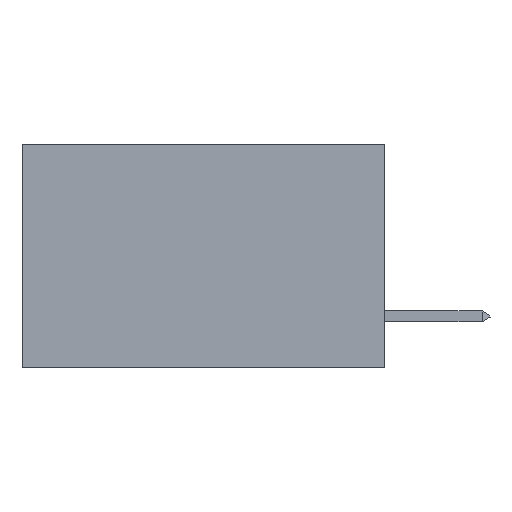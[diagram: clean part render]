
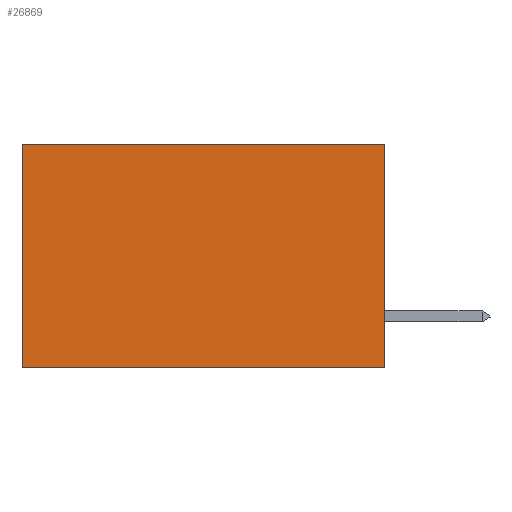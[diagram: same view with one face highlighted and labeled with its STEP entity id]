
A CAD part, left-side view. The second image highlights one B-rep face of the part: STEP entity #26869.
In plain terms, the highlighted planar face has unit normal (-1, 0, 0).
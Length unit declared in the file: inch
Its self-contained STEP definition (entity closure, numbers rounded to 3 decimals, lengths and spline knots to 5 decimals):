
#225 = DIRECTION ( 'NONE',  ( 0., 0., -1. ) ) ;
#1280 = EDGE_CURVE ( 'NONE', #16097, #14476, #20388, .T. ) ;
#3102 = AXIS2_PLACEMENT_3D ( 'NONE', #13762, #8518, #21834 ) ;
#3413 = ORIENTED_EDGE ( 'NONE', *, *, #26598, .F. ) ;
#3773 = VERTEX_POINT ( 'NONE', #14727 ) ;
#5436 = DIRECTION ( 'NONE',  ( 0., 1., 0. ) ) ;
#5950 = VECTOR ( 'NONE', #17561, 39.37008 ) ;
#6712 = CARTESIAN_POINT ( 'NONE',  ( 0.2875, 0., 0. ) ) ;
#8518 = DIRECTION ( 'NONE',  ( 1., 0., 0. ) ) ;
#9449 = VERTEX_POINT ( 'NONE', #11597 ) ;
#9648 = CARTESIAN_POINT ( 'NONE',  ( 0.2875, 0., 0. ) ) ;
#10932 = CARTESIAN_POINT ( 'NONE',  ( 0.2875, 0.6, -0.37 ) ) ;
#11597 = CARTESIAN_POINT ( 'NONE',  ( 0.2875, 0., -0.37 ) ) ;
#13762 = CARTESIAN_POINT ( 'NONE',  ( 0.2875, 0., 0. ) ) ;
#14197 = VECTOR ( 'NONE', #5436, 39.37008 ) ;
#14476 = VERTEX_POINT ( 'NONE', #10932 ) ;
#14727 = CARTESIAN_POINT ( 'NONE',  ( 0.2875, 0., 0. ) ) ;
#15000 = ORIENTED_EDGE ( 'NONE', *, *, #15804, .F. ) ;
#15804 = EDGE_CURVE ( 'NONE', #9449, #14476, #27798, .T. ) ;
#15836 = EDGE_LOOP ( 'NONE', ( #24039, #15000, #3413, #19731 ) ) ;
#16097 = VERTEX_POINT ( 'NONE', #24825 ) ;
#16162 = FACE_OUTER_BOUND ( 'NONE', #15836, .T. ) ;
#16618 = VECTOR ( 'NONE', #225, 39.37008 ) ;
#17561 = DIRECTION ( 'NONE',  ( 0., 0., -1. ) ) ;
#18819 = PLANE ( 'NONE',  #3102 ) ;
#18842 = EDGE_CURVE ( 'NONE', #3773, #16097, #23104, .T. ) ;
#19731 = ORIENTED_EDGE ( 'NONE', *, *, #18842, .T. ) ;
#20388 = LINE ( 'NONE', #33417, #16618 ) ;
#21169 = CARTESIAN_POINT ( 'NONE',  ( 0.2875, 0., -0.37 ) ) ;
#21834 = DIRECTION ( 'NONE',  ( 0., 0., -1. ) ) ;
#22083 = DIRECTION ( 'NONE',  ( 0., 1., 0. ) ) ;
#23104 = LINE ( 'NONE', #6712, #25132 ) ;
#24039 = ORIENTED_EDGE ( 'NONE', *, *, #1280, .T. ) ;
#24825 = CARTESIAN_POINT ( 'NONE',  ( 0.2875, 0.6, 0. ) ) ;
#25132 = VECTOR ( 'NONE', #22083, 39.37008 ) ;
#26429 = LINE ( 'NONE', #9648, #5950 ) ;
#26598 = EDGE_CURVE ( 'NONE', #3773, #9449, #26429, .T. ) ;
#26869 = ADVANCED_FACE ( 'NONE', ( #16162 ), #18819, .F. ) ;
#27798 = LINE ( 'NONE', #21169, #14197 ) ;
#33417 = CARTESIAN_POINT ( 'NONE',  ( 0.2875, 0.6, 0. ) ) ;
